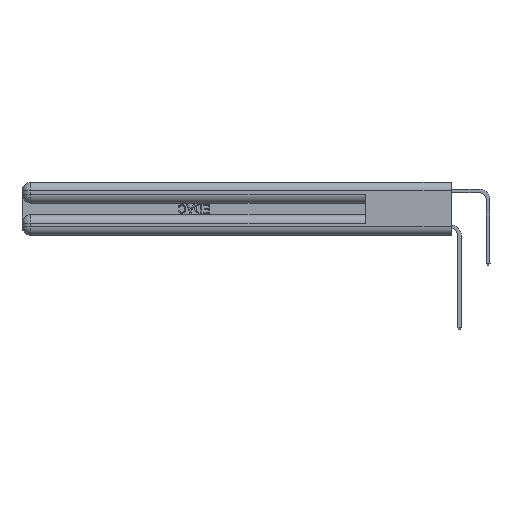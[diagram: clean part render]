
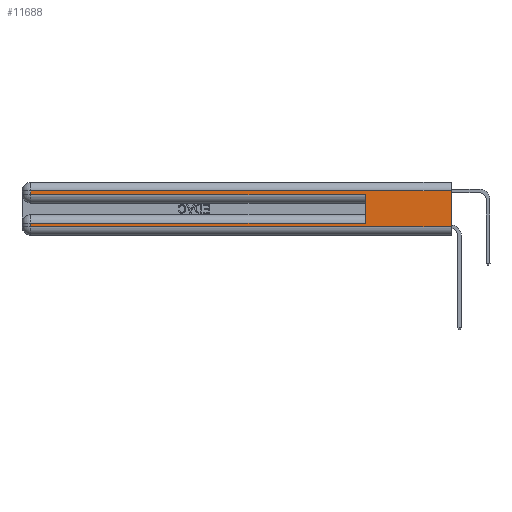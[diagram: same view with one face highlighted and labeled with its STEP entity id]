
A CAD part, left-side view. The second image highlights one B-rep face of the part: STEP entity #11688.
In plain terms, the highlighted planar face has unit normal (-1, 0, 0).
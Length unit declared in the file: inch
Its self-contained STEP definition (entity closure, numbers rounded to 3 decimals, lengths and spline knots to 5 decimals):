
#78 = ORIENTED_EDGE ( 'NONE', *, *, #7873, .T. ) ;
#906 = VERTEX_POINT ( 'NONE', #22602 ) ;
#2266 = VERTEX_POINT ( 'NONE', #3693 ) ;
#2943 = EDGE_CURVE ( 'NONE', #27612, #21330, #20244, .T. ) ;
#3113 = EDGE_CURVE ( 'NONE', #3963, #31146, #8406, .T. ) ;
#3376 = VECTOR ( 'NONE', #27587, 39.37008 ) ;
#3693 = CARTESIAN_POINT ( 'NONE',  ( 0., 0.6, 0.085 ) ) ;
#3963 = VERTEX_POINT ( 'NONE', #16293 ) ;
#4446 = CARTESIAN_POINT ( 'NONE',  ( 0., 2.94, 0.285 ) ) ;
#4858 = ORIENTED_EDGE ( 'NONE', *, *, #5105, .T. ) ;
#4930 = LINE ( 'NONE', #24801, #17342 ) ;
#4942 = CARTESIAN_POINT ( 'NONE',  ( 0., 0., 0.285 ) ) ;
#4985 = CARTESIAN_POINT ( 'NONE',  ( 0., 0.6, 0.285 ) ) ;
#5105 = EDGE_CURVE ( 'NONE', #2266, #906, #4930, .T. ) ;
#5325 = DIRECTION ( 'NONE',  ( 0., -1., 0. ) ) ;
#6974 = ORIENTED_EDGE ( 'NONE', *, *, #23594, .T. ) ;
#7067 = CARTESIAN_POINT ( 'NONE',  ( 0., 2.94, 0.37 ) ) ;
#7406 = ORIENTED_EDGE ( 'NONE', *, *, #20562, .F. ) ;
#7639 = AXIS2_PLACEMENT_3D ( 'NONE', #10842, #25524, #13454 ) ;
#7659 = LINE ( 'NONE', #17593, #27077 ) ;
#7873 = EDGE_CURVE ( 'NONE', #8079, #10503, #29255, .T. ) ;
#8021 = EDGE_CURVE ( 'NONE', #906, #3963, #17979, .T. ) ;
#8079 = VERTEX_POINT ( 'NONE', #12758 ) ;
#8406 = LINE ( 'NONE', #15419, #26183 ) ;
#9977 = DIRECTION ( 'NONE',  ( 0., 1., 0. ) ) ;
#10317 = DIRECTION ( 'NONE',  ( 0., 0., -1. ) ) ;
#10503 = VERTEX_POINT ( 'NONE', #31220 ) ;
#10794 = DIRECTION ( 'NONE',  ( 0., 0., -1. ) ) ;
#10842 = CARTESIAN_POINT ( 'NONE',  ( 0., 0., 0.37 ) ) ;
#11688 = ADVANCED_FACE ( 'NONE', ( #20645 ), #25859, .F. ) ;
#12270 = ORIENTED_EDGE ( 'NONE', *, *, #17271, .F. ) ;
#12758 = CARTESIAN_POINT ( 'NONE',  ( 0., 0., 0.31 ) ) ;
#12763 = ORIENTED_EDGE ( 'NONE', *, *, #8021, .T. ) ;
#13259 = VECTOR ( 'NONE', #10317, 39.37008 ) ;
#13454 = DIRECTION ( 'NONE',  ( 0., 0., -1. ) ) ;
#15419 = CARTESIAN_POINT ( 'NONE',  ( 0., 0., 0.06 ) ) ;
#16293 = CARTESIAN_POINT ( 'NONE',  ( 0., 2.94, 0.06 ) ) ;
#16834 = DIRECTION ( 'NONE',  ( 0., 1., 0. ) ) ;
#17000 = DIRECTION ( 'NONE',  ( 0., 0., -1. ) ) ;
#17271 = EDGE_CURVE ( 'NONE', #8079, #31146, #20749, .T. ) ;
#17342 = VECTOR ( 'NONE', #9977, 39.37008 ) ;
#17593 = CARTESIAN_POINT ( 'NONE',  ( 0., 0.6, 0.145 ) ) ;
#17979 = LINE ( 'NONE', #20739, #13259 ) ;
#20244 = LINE ( 'NONE', #4942, #3376 ) ;
#20562 = EDGE_CURVE ( 'NONE', #2266, #21330, #7659, .T. ) ;
#20645 = FACE_OUTER_BOUND ( 'NONE', #27299, .T. ) ;
#20739 = CARTESIAN_POINT ( 'NONE',  ( 0., 2.94, 0.37 ) ) ;
#20749 = LINE ( 'NONE', #21079, #31256 ) ;
#21079 = CARTESIAN_POINT ( 'NONE',  ( 0., 0., 0.37 ) ) ;
#21330 = VERTEX_POINT ( 'NONE', #4985 ) ;
#22602 = CARTESIAN_POINT ( 'NONE',  ( 0., 2.94, 0.085 ) ) ;
#22966 = DIRECTION ( 'NONE',  ( 0., 0., 1. ) ) ;
#23032 = VECTOR ( 'NONE', #17000, 39.37008 ) ;
#23594 = EDGE_CURVE ( 'NONE', #10503, #27612, #29419, .T. ) ;
#24801 = CARTESIAN_POINT ( 'NONE',  ( 0., 0., 0.085 ) ) ;
#25524 = DIRECTION ( 'NONE',  ( 1., 0., 0. ) ) ;
#25859 = PLANE ( 'NONE',  #7639 ) ;
#26075 = ORIENTED_EDGE ( 'NONE', *, *, #2943, .T. ) ;
#26183 = VECTOR ( 'NONE', #5325, 39.37008 ) ;
#26810 = VECTOR ( 'NONE', #16834, 39.37008 ) ;
#27077 = VECTOR ( 'NONE', #22966, 39.37008 ) ;
#27299 = EDGE_LOOP ( 'NONE', ( #12270, #78, #6974, #26075, #7406, #4858, #12763, #32056 ) ) ;
#27587 = DIRECTION ( 'NONE',  ( 0., -1., 0. ) ) ;
#27612 = VERTEX_POINT ( 'NONE', #4446 ) ;
#28073 = CARTESIAN_POINT ( 'NONE',  ( 0., 0., 0.06 ) ) ;
#29255 = LINE ( 'NONE', #31881, #26810 ) ;
#29419 = LINE ( 'NONE', #7067, #23032 ) ;
#31146 = VERTEX_POINT ( 'NONE', #28073 ) ;
#31220 = CARTESIAN_POINT ( 'NONE',  ( 0., 2.94, 0.31 ) ) ;
#31256 = VECTOR ( 'NONE', #10794, 39.37008 ) ;
#31881 = CARTESIAN_POINT ( 'NONE',  ( 0., 0., 0.31 ) ) ;
#32056 = ORIENTED_EDGE ( 'NONE', *, *, #3113, .T. ) ;
